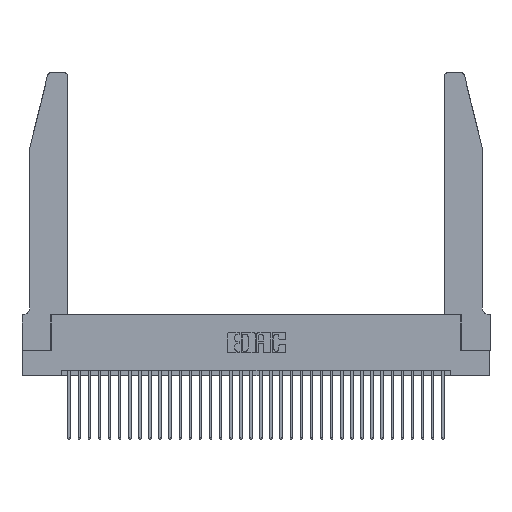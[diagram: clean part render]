
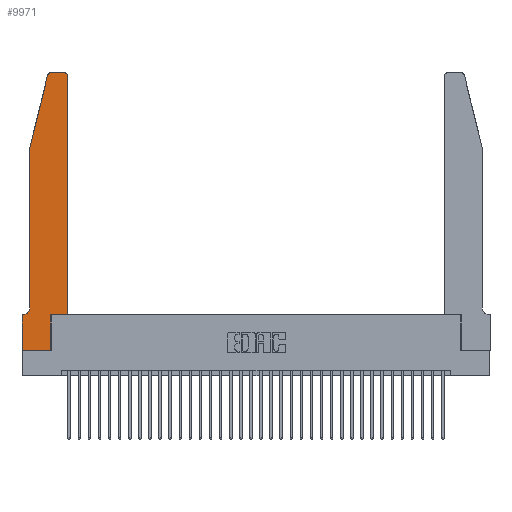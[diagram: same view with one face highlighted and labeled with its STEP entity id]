
A CAD part, top view. The second image highlights one B-rep face of the part: STEP entity #9971.
In plain terms, the highlighted planar face has unit normal (0, 0, 1).
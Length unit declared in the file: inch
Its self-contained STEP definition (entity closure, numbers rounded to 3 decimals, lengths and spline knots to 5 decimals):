
#95 = VERTEX_POINT ( 'NONE', #26453 ) ;
#336 = CARTESIAN_POINT ( 'NONE',  ( 0.4505, 0.35, 0.37 ) ) ;
#677 = CARTESIAN_POINT ( 'NONE',  ( 0.2865, 0.35, 0.37 ) ) ;
#746 = DIRECTION ( 'NONE',  ( 0., 1., 0. ) ) ;
#814 = DIRECTION ( 'NONE',  ( -1., 0., 0. ) ) ;
#853 = ORIENTED_EDGE ( 'NONE', *, *, #17902, .T. ) ;
#1261 = DIRECTION ( 'NONE',  ( -0.239, -0.971, 0. ) ) ;
#1419 = ORIENTED_EDGE ( 'NONE', *, *, #24997, .T. ) ;
#1945 = ORIENTED_EDGE ( 'NONE', *, *, #29364, .T. ) ;
#2297 = EDGE_CURVE ( 'NONE', #12227, #24888, #14900, .T. ) ;
#2370 = DIRECTION ( 'NONE',  ( 1., 0., 0. ) ) ;
#2395 = ORIENTED_EDGE ( 'NONE', *, *, #26046, .T. ) ;
#2461 = ORIENTED_EDGE ( 'NONE', *, *, #4235, .T. ) ;
#3034 = VERTEX_POINT ( 'NONE', #3364 ) ;
#3147 = CARTESIAN_POINT ( 'NONE',  ( 0.4505, 0.35, 0.37 ) ) ;
#3224 = VERTEX_POINT ( 'NONE', #3737 ) ;
#3246 = VERTEX_POINT ( 'NONE', #33464 ) ;
#3285 = VERTEX_POINT ( 'NONE', #33806 ) ;
#3364 = CARTESIAN_POINT ( 'NONE',  ( 0.2865, 0.35, 0.37 ) ) ;
#3663 = LINE ( 'NONE', #3147, #17690 ) ;
#3737 = CARTESIAN_POINT ( 'NONE',  ( 0.25487, 2.72718, 0.37 ) ) ;
#3945 = VERTEX_POINT ( 'NONE', #6379 ) ;
#4102 = LINE ( 'NONE', #19653, #26727 ) ;
#4168 = EDGE_CURVE ( 'NONE', #3246, #18927, #23773, .T. ) ;
#4235 = EDGE_CURVE ( 'NONE', #14006, #3945, #4102, .T. ) ;
#4487 = CARTESIAN_POINT ( 'NONE',  ( 0.0055, 0.42, 0.37 ) ) ;
#5211 = LINE ( 'NONE', #27584, #29930 ) ;
#5807 = VERTEX_POINT ( 'NONE', #11078 ) ;
#5889 = DIRECTION ( 'NONE',  ( 1., 0., 0. ) ) ;
#6065 = CARTESIAN_POINT ( 'NONE',  ( 0.4505, 0.35, 0.37 ) ) ;
#6379 = CARTESIAN_POINT ( 'NONE',  ( 0., 0., 0.37 ) ) ;
#6687 = CARTESIAN_POINT ( 'NONE',  ( 0.4205, 2.75, 0.37 ) ) ;
#7267 = LINE ( 'NONE', #677, #17912 ) ;
#7638 = EDGE_CURVE ( 'NONE', #24888, #3285, #32939, .T. ) ;
#7870 = LINE ( 'NONE', #9816, #9106 ) ;
#8592 = DIRECTION ( 'NONE',  ( 1., 0., 0. ) ) ;
#8799 = ORIENTED_EDGE ( 'NONE', *, *, #10167, .T. ) ;
#9106 = VECTOR ( 'NONE', #12582, 39.37008 ) ;
#9816 = CARTESIAN_POINT ( 'NONE',  ( 0., 0., 0.37 ) ) ;
#9869 = ORIENTED_EDGE ( 'NONE', *, *, #28633, .T. ) ;
#9941 = DIRECTION ( 'NONE',  ( -1., 0., 0. ) ) ;
#9971 = ADVANCED_FACE ( 'NONE', ( #15395 ), #10331, .T. ) ;
#10167 = EDGE_CURVE ( 'NONE', #5807, #3034, #7267, .T. ) ;
#10230 = CARTESIAN_POINT ( 'NONE',  ( 0.284, 2.72, 0.37 ) ) ;
#10331 = PLANE ( 'NONE',  #17601 ) ;
#10586 = LINE ( 'NONE', #6065, #16124 ) ;
#11078 = CARTESIAN_POINT ( 'NONE',  ( 0.2865, 0., 0.37 ) ) ;
#11472 = EDGE_LOOP ( 'NONE', ( #15243, #1419, #2395, #31327, #19636, #1945, #2461, #23928, #8799, #853, #9869, #19312 ) ) ;
#12179 = CARTESIAN_POINT ( 'NONE',  ( 0.4505, 2.72, 0.37 ) ) ;
#12227 = VERTEX_POINT ( 'NONE', #12179 ) ;
#12582 = DIRECTION ( 'NONE',  ( 1., 0., 0. ) ) ;
#14006 = VERTEX_POINT ( 'NONE', #22822 ) ;
#14900 = CIRCLE ( 'NONE', #21112, 0.03 ) ;
#15243 = ORIENTED_EDGE ( 'NONE', *, *, #7638, .T. ) ;
#15395 = FACE_OUTER_BOUND ( 'NONE', #11472, .T. ) ;
#16124 = VECTOR ( 'NONE', #746, 39.37008 ) ;
#16821 = CARTESIAN_POINT ( 'NONE',  ( 0.0755, 2., 0.37 ) ) ;
#17200 = CARTESIAN_POINT ( 'NONE',  ( 0.0755, 0.35, 0.37 ) ) ;
#17601 = AXIS2_PLACEMENT_3D ( 'NONE', #21642, #24433, #5889 ) ;
#17690 = VECTOR ( 'NONE', #8592, 39.37008 ) ;
#17902 = EDGE_CURVE ( 'NONE', #3034, #21743, #3663, .T. ) ;
#17912 = VECTOR ( 'NONE', #28164, 39.37008 ) ;
#18429 = EDGE_CURVE ( 'NONE', #3945, #5807, #7870, .T. ) ;
#18635 = CARTESIAN_POINT ( 'NONE',  ( 0.4205, 2.72, 0.37 ) ) ;
#18927 = VERTEX_POINT ( 'NONE', #27918 ) ;
#19312 = ORIENTED_EDGE ( 'NONE', *, *, #2297, .T. ) ;
#19636 = ORIENTED_EDGE ( 'NONE', *, *, #4168, .T. ) ;
#19653 = CARTESIAN_POINT ( 'NONE',  ( 0., 0., 0.37 ) ) ;
#20338 = VECTOR ( 'NONE', #814, 39.37008 ) ;
#20712 = VECTOR ( 'NONE', #1261, 39.37008 ) ;
#21112 = AXIS2_PLACEMENT_3D ( 'NONE', #18635, #21275, #2370 ) ;
#21187 = LINE ( 'NONE', #17200, #20338 ) ;
#21275 = DIRECTION ( 'NONE',  ( 0., 0., 1. ) ) ;
#21642 = CARTESIAN_POINT ( 'NONE',  ( 0., 0.35, 0.37 ) ) ;
#21743 = VERTEX_POINT ( 'NONE', #336 ) ;
#22822 = CARTESIAN_POINT ( 'NONE',  ( 0., 0.35, 0.37 ) ) ;
#23630 = DIRECTION ( 'NONE',  ( -1., 0., 0. ) ) ;
#23773 = CIRCLE ( 'NONE', #28028, 0.07 ) ;
#23928 = ORIENTED_EDGE ( 'NONE', *, *, #18429, .T. ) ;
#24433 = DIRECTION ( 'NONE',  ( 0., 0., 1. ) ) ;
#24750 = AXIS2_PLACEMENT_3D ( 'NONE', #10230, #29070, #34261 ) ;
#24888 = VERTEX_POINT ( 'NONE', #6687 ) ;
#24997 = EDGE_CURVE ( 'NONE', #3285, #3224, #32650, .T. ) ;
#25794 = VECTOR ( 'NONE', #23630, 39.37008 ) ;
#26023 = DIRECTION ( 'NONE',  ( 0., -1., 0. ) ) ;
#26046 = EDGE_CURVE ( 'NONE', #3224, #95, #33419, .T. ) ;
#26453 = CARTESIAN_POINT ( 'NONE',  ( 0.0755, 2., 0.37 ) ) ;
#26727 = VECTOR ( 'NONE', #26023, 39.37008 ) ;
#27240 = DIRECTION ( 'NONE',  ( 0., -1., 0. ) ) ;
#27584 = CARTESIAN_POINT ( 'NONE',  ( 0.0755, 2., 0.37 ) ) ;
#27918 = CARTESIAN_POINT ( 'NONE',  ( 0.0055, 0.35, 0.37 ) ) ;
#28028 = AXIS2_PLACEMENT_3D ( 'NONE', #4487, #28667, #9941 ) ;
#28164 = DIRECTION ( 'NONE',  ( 0., 1., 0. ) ) ;
#28633 = EDGE_CURVE ( 'NONE', #21743, #12227, #10586, .T. ) ;
#28667 = DIRECTION ( 'NONE',  ( 0., 0., -1. ) ) ;
#29070 = DIRECTION ( 'NONE',  ( 0., 0., 1. ) ) ;
#29364 = EDGE_CURVE ( 'NONE', #18927, #14006, #21187, .T. ) ;
#29930 = VECTOR ( 'NONE', #27240, 39.37008 ) ;
#31327 = ORIENTED_EDGE ( 'NONE', *, *, #34662, .T. ) ;
#31672 = CARTESIAN_POINT ( 'NONE',  ( 0.2605, 2.75, 0.37 ) ) ;
#32650 = CIRCLE ( 'NONE', #24750, 0.03 ) ;
#32939 = LINE ( 'NONE', #31672, #25794 ) ;
#33419 = LINE ( 'NONE', #16821, #20712 ) ;
#33464 = CARTESIAN_POINT ( 'NONE',  ( 0.0755, 0.42, 0.37 ) ) ;
#33806 = CARTESIAN_POINT ( 'NONE',  ( 0.284, 2.75, 0.37 ) ) ;
#34261 = DIRECTION ( 'NONE',  ( 1., 0., 0. ) ) ;
#34662 = EDGE_CURVE ( 'NONE', #95, #3246, #5211, .T. ) ;
